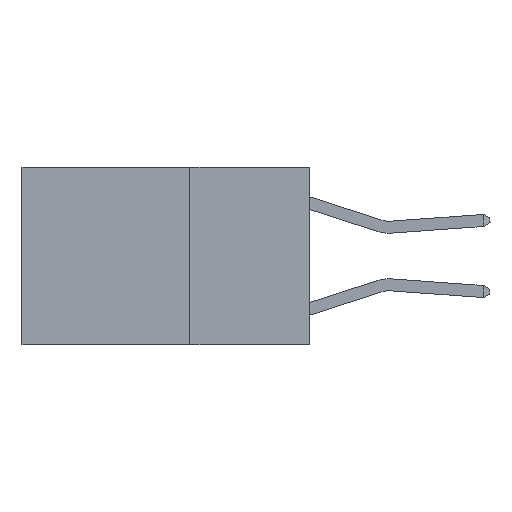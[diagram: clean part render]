
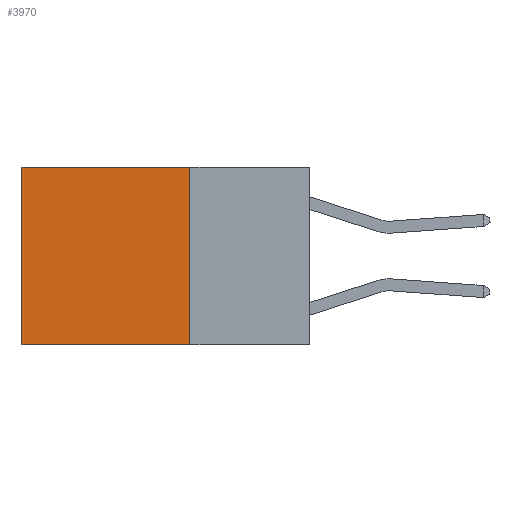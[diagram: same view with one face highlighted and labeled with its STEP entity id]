
A CAD part, left-side view. The second image highlights one B-rep face of the part: STEP entity #3970.
In plain terms, the highlighted planar face has unit normal (-1, 0, 0).
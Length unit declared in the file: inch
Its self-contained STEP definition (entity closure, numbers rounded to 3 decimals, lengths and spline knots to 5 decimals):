
#194 = CARTESIAN_POINT ( 'NONE',  ( 0.2625, 0.25, 0. ) ) ;
#462 = DIRECTION ( 'NONE',  ( 0., 1., 0. ) ) ;
#771 = EDGE_CURVE ( 'NONE', #7987, #9464, #1127, .T. ) ;
#1127 = LINE ( 'NONE', #7316, #7096 ) ;
#1262 = DIRECTION ( 'NONE',  ( 0., 1., 0. ) ) ;
#1414 = CARTESIAN_POINT ( 'NONE',  ( 0.2625, 0.25, 0. ) ) ;
#1529 = CARTESIAN_POINT ( 'NONE',  ( 0.2625, 0.6, 0. ) ) ;
#2433 = ORIENTED_EDGE ( 'NONE', *, *, #771, .F. ) ;
#2524 = LINE ( 'NONE', #1529, #13093 ) ;
#2598 = CARTESIAN_POINT ( 'NONE',  ( 0.2625, 0.25, -0.37 ) ) ;
#2940 = DIRECTION ( 'NONE',  ( 0., 0., -1. ) ) ;
#3111 = LINE ( 'NONE', #194, #11206 ) ;
#3138 = VERTEX_POINT ( 'NONE', #3758 ) ;
#3565 = LINE ( 'NONE', #2598, #10999 ) ;
#3651 = VERTEX_POINT ( 'NONE', #4595 ) ;
#3758 = CARTESIAN_POINT ( 'NONE',  ( 0.2625, 0.6, 0. ) ) ;
#3929 = ORIENTED_EDGE ( 'NONE', *, *, #8556, .T. ) ;
#3970 = ADVANCED_FACE ( 'NONE', ( #8011 ), #13448, .F. ) ;
#4387 = EDGE_LOOP ( 'NONE', ( #11109, #5513, #2433, #3929 ) ) ;
#4595 = CARTESIAN_POINT ( 'NONE',  ( 0.2625, 0.6, -0.37 ) ) ;
#5513 = ORIENTED_EDGE ( 'NONE', *, *, #10562, .F. ) ;
#7096 = VECTOR ( 'NONE', #13594, 39.37008 ) ;
#7316 = CARTESIAN_POINT ( 'NONE',  ( 0.2625, 0.25, 0. ) ) ;
#7987 = VERTEX_POINT ( 'NONE', #1414 ) ;
#8011 = FACE_OUTER_BOUND ( 'NONE', #4387, .T. ) ;
#8556 = EDGE_CURVE ( 'NONE', #7987, #3138, #3111, .T. ) ;
#8586 = AXIS2_PLACEMENT_3D ( 'NONE', #11350, #9301, #2940 ) ;
#9261 = CARTESIAN_POINT ( 'NONE',  ( 0.2625, 0.25, -0.37 ) ) ;
#9301 = DIRECTION ( 'NONE',  ( 1., 0., 0. ) ) ;
#9464 = VERTEX_POINT ( 'NONE', #9261 ) ;
#10562 = EDGE_CURVE ( 'NONE', #9464, #3651, #3565, .T. ) ;
#10999 = VECTOR ( 'NONE', #462, 39.37008 ) ;
#11109 = ORIENTED_EDGE ( 'NONE', *, *, #12249, .T. ) ;
#11206 = VECTOR ( 'NONE', #1262, 39.37008 ) ;
#11350 = CARTESIAN_POINT ( 'NONE',  ( 0.2625, 0.25, 0. ) ) ;
#12249 = EDGE_CURVE ( 'NONE', #3138, #3651, #2524, .T. ) ;
#13093 = VECTOR ( 'NONE', #13112, 39.37008 ) ;
#13112 = DIRECTION ( 'NONE',  ( 0., 0., -1. ) ) ;
#13448 = PLANE ( 'NONE',  #8586 ) ;
#13594 = DIRECTION ( 'NONE',  ( 0., 0., -1. ) ) ;
